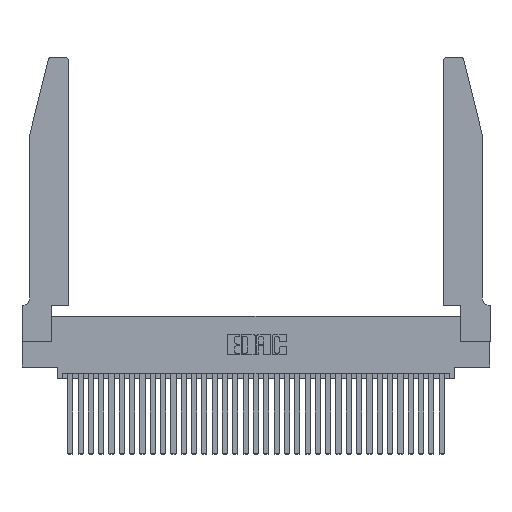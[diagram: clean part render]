
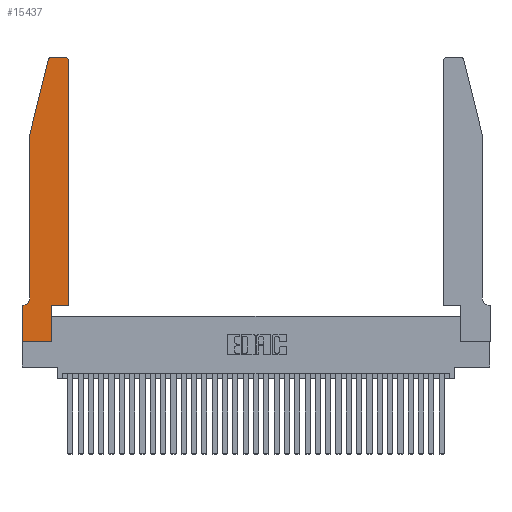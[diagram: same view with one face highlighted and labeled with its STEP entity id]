
A CAD part, top view. The second image highlights one B-rep face of the part: STEP entity #15437.
In plain terms, the highlighted planar face has unit normal (0, 0, 1).
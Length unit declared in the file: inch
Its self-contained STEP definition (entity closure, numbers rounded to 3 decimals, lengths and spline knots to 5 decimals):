
#108 = VECTOR ( 'NONE', #26030, 39.37008 ) ;
#1040 = LINE ( 'NONE', #34036, #17330 ) ;
#1373 = LINE ( 'NONE', #29366, #30592 ) ;
#2021 = LINE ( 'NONE', #7865, #20799 ) ;
#2120 = CARTESIAN_POINT ( 'NONE',  ( 0.4205, 2.75, 0.37 ) ) ;
#2325 = ORIENTED_EDGE ( 'NONE', *, *, #5318, .T. ) ;
#2435 = CARTESIAN_POINT ( 'NONE',  ( 0.284, 2.72, 0.37 ) ) ;
#3046 = VERTEX_POINT ( 'NONE', #21838 ) ;
#3135 = DIRECTION ( 'NONE',  ( 0., -1., 0. ) ) ;
#3634 = CARTESIAN_POINT ( 'NONE',  ( 0., 0.35, 0.37 ) ) ;
#3684 = ORIENTED_EDGE ( 'NONE', *, *, #19083, .T. ) ;
#3780 = CARTESIAN_POINT ( 'NONE',  ( 0.25487, 2.72718, 0.37 ) ) ;
#5056 = DIRECTION ( 'NONE',  ( 0., 1., 0. ) ) ;
#5318 = EDGE_CURVE ( 'NONE', #27717, #10563, #17860, .T. ) ;
#5974 = CARTESIAN_POINT ( 'NONE',  ( 0.284, 2.75, 0.37 ) ) ;
#6270 = EDGE_CURVE ( 'NONE', #22033, #25660, #2021, .T. ) ;
#6322 = DIRECTION ( 'NONE',  ( -1., 0., 0. ) ) ;
#6419 = ORIENTED_EDGE ( 'NONE', *, *, #10506, .T. ) ;
#6501 = DIRECTION ( 'NONE',  ( 0., -1., 0. ) ) ;
#7079 = CIRCLE ( 'NONE', #32345, 0.03 ) ;
#7105 = CARTESIAN_POINT ( 'NONE',  ( 0.0055, 0.42, 0.37 ) ) ;
#7499 = ORIENTED_EDGE ( 'NONE', *, *, #12031, .T. ) ;
#7865 = CARTESIAN_POINT ( 'NONE',  ( 0.0755, 2., 0.37 ) ) ;
#8010 = CARTESIAN_POINT ( 'NONE',  ( 0.0755, 2., 0.37 ) ) ;
#8080 = VECTOR ( 'NONE', #6322, 39.37008 ) ;
#8185 = DIRECTION ( 'NONE',  ( -0.239, -0.971, 0. ) ) ;
#8336 = CARTESIAN_POINT ( 'NONE',  ( 0.4505, 0.35, 0.37 ) ) ;
#8554 = CARTESIAN_POINT ( 'NONE',  ( 0.0755, 2., 0.37 ) ) ;
#8653 = CIRCLE ( 'NONE', #12772, 0.03 ) ;
#8968 = CARTESIAN_POINT ( 'NONE',  ( 0.2605, 2.75, 0.37 ) ) ;
#10016 = CARTESIAN_POINT ( 'NONE',  ( 0.4505, 0.35, 0.37 ) ) ;
#10172 = AXIS2_PLACEMENT_3D ( 'NONE', #3634, #25206, #27878 ) ;
#10335 = EDGE_LOOP ( 'NONE', ( #13739, #10652, #16529, #19802, #6419, #16351, #2325, #16330, #3684, #20164, #17221, #7499 ) ) ;
#10506 = EDGE_CURVE ( 'NONE', #26163, #3046, #20963, .T. ) ;
#10563 = VERTEX_POINT ( 'NONE', #15254 ) ;
#10652 = ORIENTED_EDGE ( 'NONE', *, *, #11733, .T. ) ;
#11523 = CARTESIAN_POINT ( 'NONE',  ( 0.4205, 2.72, 0.37 ) ) ;
#11733 = EDGE_CURVE ( 'NONE', #21753, #22033, #7079, .T. ) ;
#12031 = EDGE_CURVE ( 'NONE', #17745, #30550, #8653, .T. ) ;
#12543 = CARTESIAN_POINT ( 'NONE',  ( 0., 0.35, 0.37 ) ) ;
#12772 = AXIS2_PLACEMENT_3D ( 'NONE', #11523, #27502, #27621 ) ;
#13358 = DIRECTION ( 'NONE',  ( 1., 0., 0. ) ) ;
#13393 = DIRECTION ( 'NONE',  ( -1., 0., 0. ) ) ;
#13739 = ORIENTED_EDGE ( 'NONE', *, *, #18743, .T. ) ;
#14068 = VECTOR ( 'NONE', #6501, 39.37008 ) ;
#14829 = LINE ( 'NONE', #8968, #8080 ) ;
#15254 = CARTESIAN_POINT ( 'NONE',  ( 0., 0., 0.37 ) ) ;
#15437 = ADVANCED_FACE ( 'NONE', ( #22115 ), #17138, .T. ) ;
#15720 = LINE ( 'NONE', #25289, #30746 ) ;
#16330 = ORIENTED_EDGE ( 'NONE', *, *, #28907, .T. ) ;
#16351 = ORIENTED_EDGE ( 'NONE', *, *, #24722, .T. ) ;
#16529 = ORIENTED_EDGE ( 'NONE', *, *, #6270, .T. ) ;
#16709 = CARTESIAN_POINT ( 'NONE',  ( 0.2865, 0.35, 0.37 ) ) ;
#16969 = LINE ( 'NONE', #8554, #14068 ) ;
#17082 = DIRECTION ( 'NONE',  ( 1., 0., 0. ) ) ;
#17138 = PLANE ( 'NONE',  #10172 ) ;
#17221 = ORIENTED_EDGE ( 'NONE', *, *, #23369, .T. ) ;
#17330 = VECTOR ( 'NONE', #5056, 39.37008 ) ;
#17385 = VERTEX_POINT ( 'NONE', #16709 ) ;
#17745 = VERTEX_POINT ( 'NONE', #30248 ) ;
#17798 = DIRECTION ( 'NONE',  ( 0., 0., -1. ) ) ;
#17860 = LINE ( 'NONE', #30165, #29119 ) ;
#18447 = CARTESIAN_POINT ( 'NONE',  ( 0.2865, 0., 0.37 ) ) ;
#18743 = EDGE_CURVE ( 'NONE', #30550, #21753, #14829, .T. ) ;
#19083 = EDGE_CURVE ( 'NONE', #21358, #17385, #30546, .T. ) ;
#19802 = ORIENTED_EDGE ( 'NONE', *, *, #25323, .T. ) ;
#20164 = ORIENTED_EDGE ( 'NONE', *, *, #25560, .T. ) ;
#20799 = VECTOR ( 'NONE', #8185, 39.37008 ) ;
#20963 = CIRCLE ( 'NONE', #22581, 0.07 ) ;
#21358 = VERTEX_POINT ( 'NONE', #18447 ) ;
#21753 = VERTEX_POINT ( 'NONE', #5974 ) ;
#21838 = CARTESIAN_POINT ( 'NONE',  ( 0.0055, 0.35, 0.37 ) ) ;
#22033 = VERTEX_POINT ( 'NONE', #3780 ) ;
#22115 = FACE_OUTER_BOUND ( 'NONE', #10335, .T. ) ;
#22581 = AXIS2_PLACEMENT_3D ( 'NONE', #7105, #17798, #31108 ) ;
#23369 = EDGE_CURVE ( 'NONE', #33179, #17745, #1040, .T. ) ;
#24722 = EDGE_CURVE ( 'NONE', #3046, #27717, #1373, .T. ) ;
#25206 = DIRECTION ( 'NONE',  ( 0., 0., 1. ) ) ;
#25289 = CARTESIAN_POINT ( 'NONE',  ( 0., 0., 0.37 ) ) ;
#25323 = EDGE_CURVE ( 'NONE', #25660, #26163, #16969, .T. ) ;
#25560 = EDGE_CURVE ( 'NONE', #17385, #33179, #30933, .T. ) ;
#25660 = VERTEX_POINT ( 'NONE', #8010 ) ;
#26030 = DIRECTION ( 'NONE',  ( 0., 1., 0. ) ) ;
#26163 = VERTEX_POINT ( 'NONE', #28293 ) ;
#26332 = DIRECTION ( 'NONE',  ( 1., 0., 0. ) ) ;
#26337 = DIRECTION ( 'NONE',  ( 0., 0., 1. ) ) ;
#27502 = DIRECTION ( 'NONE',  ( 0., 0., 1. ) ) ;
#27554 = VECTOR ( 'NONE', #26332, 39.37008 ) ;
#27621 = DIRECTION ( 'NONE',  ( 1., 0., 0. ) ) ;
#27717 = VERTEX_POINT ( 'NONE', #12543 ) ;
#27878 = DIRECTION ( 'NONE',  ( 1., 0., 0. ) ) ;
#28293 = CARTESIAN_POINT ( 'NONE',  ( 0.0755, 0.42, 0.37 ) ) ;
#28907 = EDGE_CURVE ( 'NONE', #10563, #21358, #15720, .T. ) ;
#29119 = VECTOR ( 'NONE', #3135, 39.37008 ) ;
#29366 = CARTESIAN_POINT ( 'NONE',  ( 0.0755, 0.35, 0.37 ) ) ;
#30165 = CARTESIAN_POINT ( 'NONE',  ( 0., 0., 0.37 ) ) ;
#30248 = CARTESIAN_POINT ( 'NONE',  ( 0.4505, 2.72, 0.37 ) ) ;
#30546 = LINE ( 'NONE', #31252, #108 ) ;
#30550 = VERTEX_POINT ( 'NONE', #2120 ) ;
#30592 = VECTOR ( 'NONE', #13393, 39.37008 ) ;
#30746 = VECTOR ( 'NONE', #17082, 39.37008 ) ;
#30933 = LINE ( 'NONE', #10016, #27554 ) ;
#31108 = DIRECTION ( 'NONE',  ( -1., 0., 0. ) ) ;
#31252 = CARTESIAN_POINT ( 'NONE',  ( 0.2865, 0.35, 0.37 ) ) ;
#32345 = AXIS2_PLACEMENT_3D ( 'NONE', #2435, #26337, #13358 ) ;
#33179 = VERTEX_POINT ( 'NONE', #8336 ) ;
#34036 = CARTESIAN_POINT ( 'NONE',  ( 0.4505, 0.35, 0.37 ) ) ;
